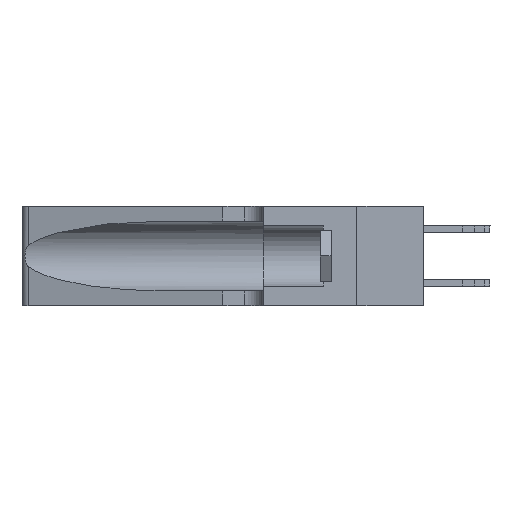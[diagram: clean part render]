
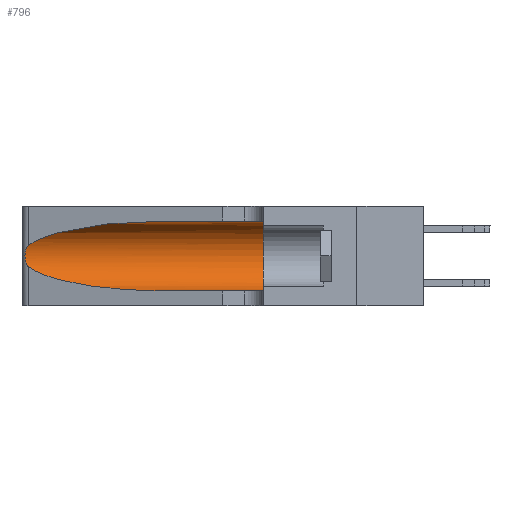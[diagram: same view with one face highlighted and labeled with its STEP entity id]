
A CAD part, left-side view. The second image highlights one B-rep face of the part: STEP entity #796.
In plain terms, the highlighted cylindrical face has radius 3.308 mm (diameter 6.617 mm), a partial arc.
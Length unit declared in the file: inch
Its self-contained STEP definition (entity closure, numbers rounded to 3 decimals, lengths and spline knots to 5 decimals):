
#434 = CARTESIAN_POINT ( 'NONE',  ( 0.25487, 1.22718, 0.14631 ) ) ;
#655 = EDGE_CURVE ( 'NONE', #8493, #9923, #13144, .T. ) ;
#796 = ADVANCED_FACE ( 'NONE', ( #7171 ), #4252, .F. ) ;
#1670 = CARTESIAN_POINT ( 'NONE',  ( 0.1305, 0.72297, 0.31525 ) ) ;
#2465 = CARTESIAN_POINT ( 'NONE',  ( 0.25856, 1.23593, 0.16098 ) ) ;
#2588 = VERTEX_POINT ( 'NONE', #10360 ) ;
#3072 = ORIENTED_EDGE ( 'NONE', *, *, #5071, .F. ) ;
#3361 = DIRECTION ( 'NONE',  ( 0., 1., 0. ) ) ;
#3505 = CARTESIAN_POINT ( 'NONE',  ( 0.2373, 1.15595, 0.08982 ) ) ;
#4202 = AXIS2_PLACEMENT_3D ( 'NONE', #10388, #19886, #16866 ) ;
#4252 = CYLINDRICAL_SURFACE ( 'NONE', #4202, 0.13025 ) ;
#4474 = ORIENTED_EDGE ( 'NONE', *, *, #655, .T. ) ;
#4695 = DIRECTION ( 'NONE',  ( 0., -1., 0. ) ) ;
#4781 = CARTESIAN_POINT ( 'NONE',  ( 0.18966, 0.96281, 0.31525 ) ) ;
#5071 = EDGE_CURVE ( 'NONE', #8493, #6684, #15331, .T. ) ;
#5332 = CARTESIAN_POINT ( 'NONE',  ( 0.1305, 0.35, 0.31525 ) ) ;
#5710 = CARTESIAN_POINT ( 'NONE',  ( 0.25787, 1.23484, 0.2124 ) ) ;
#5858 = EDGE_CURVE ( 'NONE', #2588, #14232, #8764, .T. ) ;
#6546 = DIRECTION ( 'NONE',  ( 0., -1., 0. ) ) ;
#6684 = VERTEX_POINT ( 'NONE', #5332 ) ;
#7117 = CARTESIAN_POINT ( 'NONE',  ( 0.25487, 1.22718, 0.22369 ) ) ;
#7159 = CARTESIAN_POINT ( 'NONE',  ( 0.25555, 1.22993, 0.14849 ) ) ;
#7171 = FACE_OUTER_BOUND ( 'NONE', #9584, .T. ) ;
#7467 = CARTESIAN_POINT ( 'NONE',  ( 0.1305, 0.72297, 0.31525 ) ) ;
#7675 = EDGE_CURVE ( 'NONE', #6684, #14232, #14726, .T. ) ;
#8189 = DIRECTION ( 'NONE',  ( 0., 0., 1. ) ) ;
#8322 = CARTESIAN_POINT ( 'NONE',  ( 0.2373, 1.15595, 0.28018 ) ) ;
#8493 = VERTEX_POINT ( 'NONE', #7467 ) ;
#8609 = ORIENTED_EDGE ( 'NONE', *, *, #7675, .F. ) ;
#8764 = LINE ( 'NONE', #17162, #18504 ) ;
#9584 = EDGE_LOOP ( 'NONE', ( #4474, #19206, #17810, #17817, #8609, #3072 ) ) ;
#9923 = VERTEX_POINT ( 'NONE', #14570 ) ;
#10196 = CARTESIAN_POINT ( 'NONE',  ( 0.26017, 1.23833, 0.17102 ) ) ;
#10360 = CARTESIAN_POINT ( 'NONE',  ( 0.1305, 0.72297, 0.05475 ) ) ;
#10388 = CARTESIAN_POINT ( 'NONE',  ( 0.1305, 1.61858, 0.185 ) ) ;
#10424 = B_SPLINE_CURVE_WITH_KNOTS ( 'NONE', 3,
 ( #11851, #14808, #13407, #5710, #17843, #19376, #14947, #13209, #10196, #2465, #14885, #16467, #7159, #19591 ),
 .UNSPECIFIED., .F., .F.,
 ( 4, 2, 2, 2, 2, 2, 4 ),
 ( 0., 0.00027, 0.00053, 0.00107, 0.0016, 0.00187, 0.00214 ),
 .UNSPECIFIED. ) ;
#11616 = EDGE_CURVE ( 'NONE', #15575, #2588, #11899, .T. ) ;
#11851 = CARTESIAN_POINT ( 'NONE',  ( 0.25487, 1.22718, 0.22369 ) ) ;
#11899 =( BOUNDED_CURVE ( )  B_SPLINE_CURVE ( 3, ( #434, #3505, #15951, #15679 ),
 .UNSPECIFIED., .F., .F. ) 
 B_SPLINE_CURVE_WITH_KNOTS ( ( 4, 4 ),
 ( 3.44316, 4.71239 ),
 .UNSPECIFIED. ) 
 CURVE ( )  GEOMETRIC_REPRESENTATION_ITEM ( )  RATIONAL_B_SPLINE_CURVE ( ( 1., 0.87, 0.87, 1. ) ) 
 REPRESENTATION_ITEM ( '' )  );
#12008 = CARTESIAN_POINT ( 'NONE',  ( 0.1305, 0.35, 0.05475 ) ) ;
#12851 = CARTESIAN_POINT ( 'NONE',  ( 0.1305, 0.35, 0.185 ) ) ;
#13144 =( BOUNDED_CURVE ( )  B_SPLINE_CURVE ( 3, ( #1670, #4781, #8322, #7117 ),
 .UNSPECIFIED., .F., .F. ) 
 B_SPLINE_CURVE_WITH_KNOTS ( ( 4, 4 ),
 ( 1.5708, 2.84003 ),
 .UNSPECIFIED. ) 
 CURVE ( )  GEOMETRIC_REPRESENTATION_ITEM ( )  RATIONAL_B_SPLINE_CURVE ( ( 1., 0.87, 0.87, 1. ) ) 
 REPRESENTATION_ITEM ( '' )  );
#13209 = CARTESIAN_POINT ( 'NONE',  ( 0.26075, 1.23896, 0.178 ) ) ;
#13407 = CARTESIAN_POINT ( 'NONE',  ( 0.25639, 1.23184, 0.21858 ) ) ;
#14232 = VERTEX_POINT ( 'NONE', #12008 ) ;
#14570 = CARTESIAN_POINT ( 'NONE',  ( 0.25487, 1.22718, 0.22369 ) ) ;
#14726 = CIRCLE ( 'NONE', #18747, 0.13025 ) ;
#14808 = CARTESIAN_POINT ( 'NONE',  ( 0.25555, 1.22994, 0.2215 ) ) ;
#14885 = CARTESIAN_POINT ( 'NONE',  ( 0.25789, 1.23486, 0.15765 ) ) ;
#14947 = CARTESIAN_POINT ( 'NONE',  ( 0.26075, 1.23896, 0.19203 ) ) ;
#15331 = LINE ( 'NONE', #17511, #19948 ) ;
#15354 = EDGE_CURVE ( 'NONE', #9923, #15575, #10424, .T. ) ;
#15565 = CARTESIAN_POINT ( 'NONE',  ( 0.25487, 1.22718, 0.14631 ) ) ;
#15575 = VERTEX_POINT ( 'NONE', #15565 ) ;
#15679 = CARTESIAN_POINT ( 'NONE',  ( 0.1305, 0.72297, 0.05475 ) ) ;
#15951 = CARTESIAN_POINT ( 'NONE',  ( 0.18966, 0.96281, 0.05475 ) ) ;
#16467 = CARTESIAN_POINT ( 'NONE',  ( 0.25639, 1.23186, 0.15144 ) ) ;
#16866 = DIRECTION ( 'NONE',  ( 0., 0., -1. ) ) ;
#17162 = CARTESIAN_POINT ( 'NONE',  ( 0.1305, 1.61858, 0.05475 ) ) ;
#17511 = CARTESIAN_POINT ( 'NONE',  ( 0.1305, 1.61858, 0.31525 ) ) ;
#17810 = ORIENTED_EDGE ( 'NONE', *, *, #11616, .T. ) ;
#17817 = ORIENTED_EDGE ( 'NONE', *, *, #5858, .T. ) ;
#17843 = CARTESIAN_POINT ( 'NONE',  ( 0.25854, 1.2359, 0.20912 ) ) ;
#18504 = VECTOR ( 'NONE', #4695, 39.37008 ) ;
#18747 = AXIS2_PLACEMENT_3D ( 'NONE', #12851, #3361, #8189 ) ;
#19206 = ORIENTED_EDGE ( 'NONE', *, *, #15354, .T. ) ;
#19376 = CARTESIAN_POINT ( 'NONE',  ( 0.26018, 1.23835, 0.19895 ) ) ;
#19591 = CARTESIAN_POINT ( 'NONE',  ( 0.25487, 1.22718, 0.14631 ) ) ;
#19886 = DIRECTION ( 'NONE',  ( 0., -1., 0. ) ) ;
#19948 = VECTOR ( 'NONE', #6546, 39.37008 ) ;
